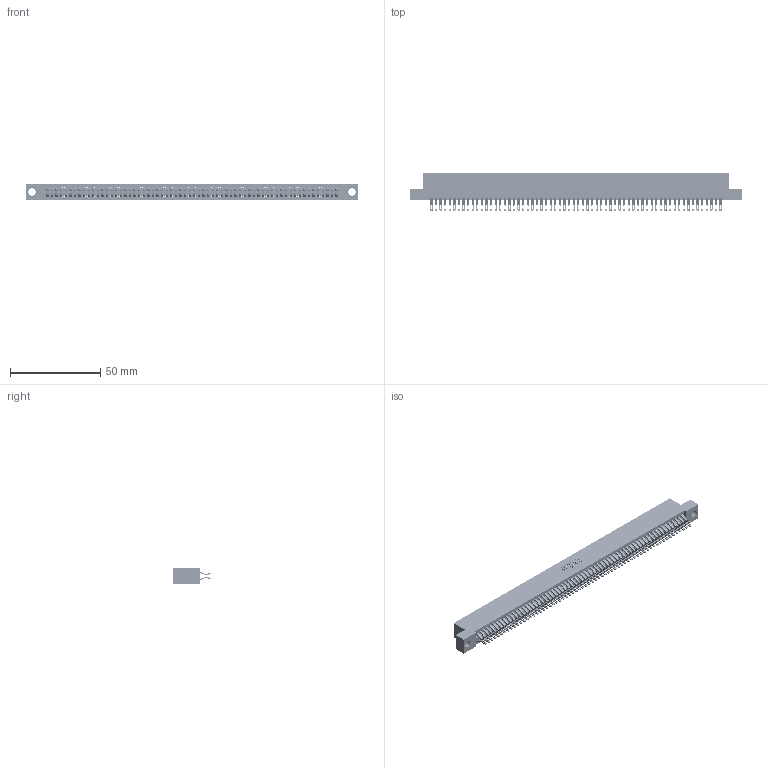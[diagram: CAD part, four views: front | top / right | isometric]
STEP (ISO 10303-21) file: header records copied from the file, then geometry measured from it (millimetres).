
FILE_DESCRIPTION (( 'STEP AP203' ), '1' );
FILE_NAME ('395-128-555-204.STEP', '2021-06-17T23:45:57', ( '' ), ( '' ), 'SwSTEP 2.0', 'SolidWorks 2020', '' );
FILE_SCHEMA (( 'CONFIG_CONTROL_DESIGN' ));
Length unit declared in the file: inch
Products named in the file (3): 395-128-555-204; 345-292-001_555 Tail; 345 Part_Flush Mounting Lugs - 0.156 Dia-TI
Assembly tree (129 placements, depth 2):
  395-128-555-204
    345 Part_Flush Mounting Lugs - 0.156 Dia-TI
    345-292-001_555 Tail  x128
Bounding box: 183.77 x 21.13 x 9.4 mm (x, y, z)
Volume: 18321 mm3; surface area: 28650.6 mm2
Topology: 129 solids, 129 shells, 7308 faces, 23033 edges, 15354 vertices
Faces by surface type: plane 4062, cylinder 3246
Entity records: 47999 total; most frequent: CARTESIAN_POINT 8064, ORIENTED_EDGE 7966, DIRECTION 7051, EDGE_CURVE 3983, VECTOR 3575, LINE 3575, VERTEX_POINT 2654, AXIS2_PLACEMENT_3D 1738
